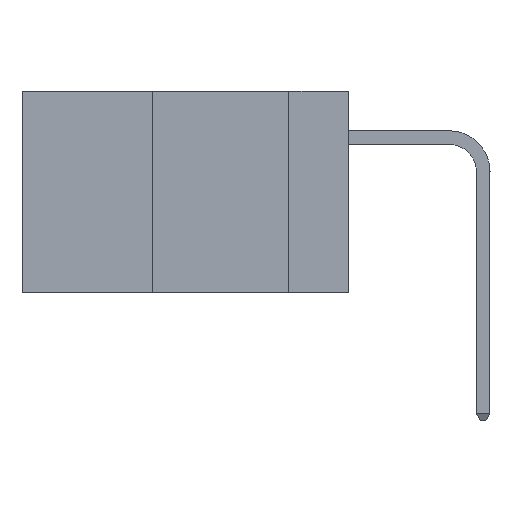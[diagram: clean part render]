
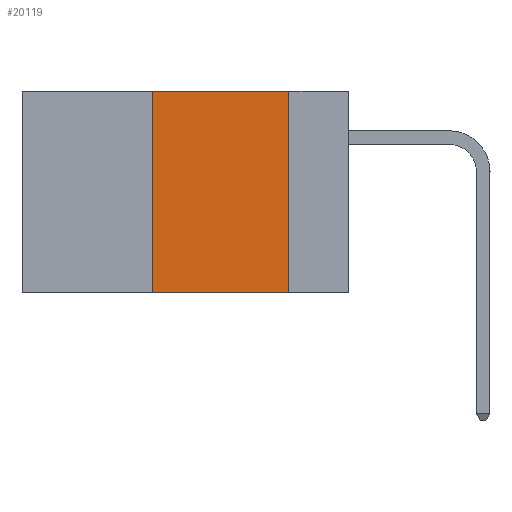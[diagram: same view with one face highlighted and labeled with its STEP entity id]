
A CAD part, left-side view. The second image highlights one B-rep face of the part: STEP entity #20119.
In plain terms, the highlighted planar face has unit normal (-1, 0, 0).
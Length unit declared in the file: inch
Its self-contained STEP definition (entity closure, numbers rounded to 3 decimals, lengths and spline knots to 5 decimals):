
#468 = CARTESIAN_POINT ( 'NONE',  ( 0., 0.36, -0.37 ) ) ;
#478 = EDGE_CURVE ( 'NONE', #22996, #4006, #28433, .T. ) ;
#863 = DIRECTION ( 'NONE',  ( 0., -1., 0. ) ) ;
#1501 = CARTESIAN_POINT ( 'NONE',  ( 0., 0.36, 0. ) ) ;
#1939 = DIRECTION ( 'NONE',  ( 0., 0., -1. ) ) ;
#2342 = FACE_OUTER_BOUND ( 'NONE', #36198, .T. ) ;
#2411 = LINE ( 'NONE', #10789, #28743 ) ;
#3613 = DIRECTION ( 'NONE',  ( 0., 0., 1. ) ) ;
#4006 = VERTEX_POINT ( 'NONE', #29241 ) ;
#6094 = VERTEX_POINT ( 'NONE', #1501 ) ;
#6729 = CARTESIAN_POINT ( 'NONE',  ( 0., 0.6, -0.37 ) ) ;
#8803 = EDGE_CURVE ( 'NONE', #16556, #6094, #26605, .T. ) ;
#9769 = DIRECTION ( 'NONE',  ( 0., 0., -1. ) ) ;
#9895 = CARTESIAN_POINT ( 'NONE',  ( 0., 0.11, 0. ) ) ;
#10789 = CARTESIAN_POINT ( 'NONE',  ( 0., 0.6, 0. ) ) ;
#12028 = EDGE_CURVE ( 'NONE', #16556, #4006, #20320, .T. ) ;
#14371 = VECTOR ( 'NONE', #863, 39.37008 ) ;
#16556 = VERTEX_POINT ( 'NONE', #468 ) ;
#17865 = PLANE ( 'NONE',  #19193 ) ;
#19193 = AXIS2_PLACEMENT_3D ( 'NONE', #27247, #36833, #1939 ) ;
#20119 = ADVANCED_FACE ( 'NONE', ( #2342 ), #17865, .F. ) ;
#20320 = LINE ( 'NONE', #6729, #14371 ) ;
#22996 = VERTEX_POINT ( 'NONE', #38082 ) ;
#23044 = ORIENTED_EDGE ( 'NONE', *, *, #12028, .T. ) ;
#24557 = ORIENTED_EDGE ( 'NONE', *, *, #25492, .F. ) ;
#25492 = EDGE_CURVE ( 'NONE', #6094, #22996, #2411, .T. ) ;
#26605 = LINE ( 'NONE', #38845, #28146 ) ;
#27247 = CARTESIAN_POINT ( 'NONE',  ( 0., 0.6, 0. ) ) ;
#28146 = VECTOR ( 'NONE', #3613, 39.37008 ) ;
#28433 = LINE ( 'NONE', #9895, #29414 ) ;
#28743 = VECTOR ( 'NONE', #40497, 39.37008 ) ;
#29241 = CARTESIAN_POINT ( 'NONE',  ( 0., 0.11, -0.37 ) ) ;
#29414 = VECTOR ( 'NONE', #9769, 39.37008 ) ;
#29498 = ORIENTED_EDGE ( 'NONE', *, *, #478, .F. ) ;
#36198 = EDGE_LOOP ( 'NONE', ( #29498, #24557, #37899, #23044 ) ) ;
#36833 = DIRECTION ( 'NONE',  ( 1., 0., 0. ) ) ;
#37899 = ORIENTED_EDGE ( 'NONE', *, *, #8803, .F. ) ;
#38082 = CARTESIAN_POINT ( 'NONE',  ( 0., 0.11, 0. ) ) ;
#38845 = CARTESIAN_POINT ( 'NONE',  ( 0., 0.36, 0. ) ) ;
#40497 = DIRECTION ( 'NONE',  ( 0., -1., 0. ) ) ;
